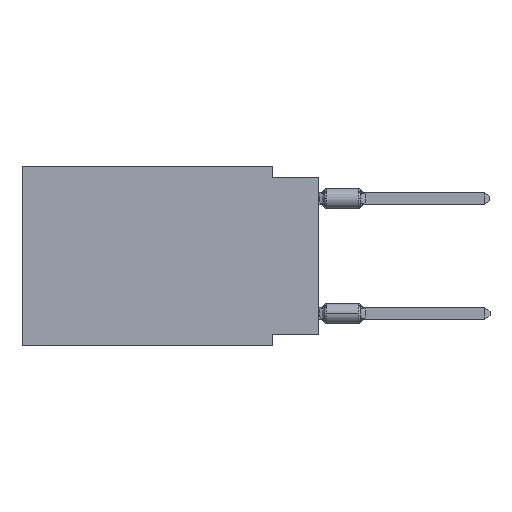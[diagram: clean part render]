
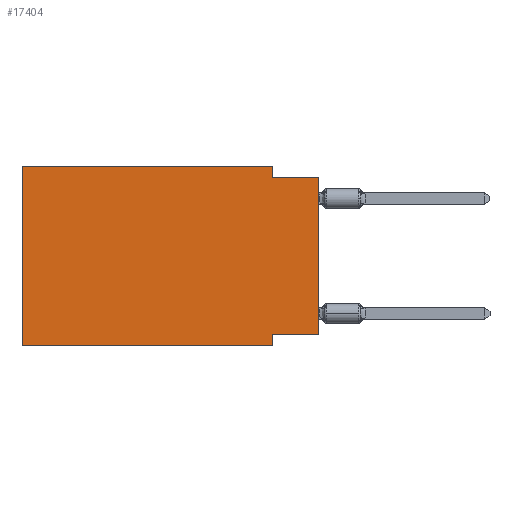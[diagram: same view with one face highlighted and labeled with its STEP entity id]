
A CAD part, left-side view. The second image highlights one B-rep face of the part: STEP entity #17404.
In plain terms, the highlighted planar face has unit normal (-1, 0, 0).
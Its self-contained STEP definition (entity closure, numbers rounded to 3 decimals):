
#373 = EDGE_CURVE ( 'NONE', #12863, #6835, #8443, .T. ) ;
#426 = VERTEX_POINT ( 'NONE', #7139 ) ;
#1110 = DIRECTION ( 'NONE',  ( 0., 0., 1. ) ) ;
#2010 = ORIENTED_EDGE ( 'NONE', *, *, #9848, .F. ) ;
#2150 = CARTESIAN_POINT ( 'NONE',  ( 0., 2.54, 0. ) ) ;
#3019 = ORIENTED_EDGE ( 'NONE', *, *, #11672, .F. ) ;
#4053 = LINE ( 'NONE', #6963, #6411 ) ;
#4659 = ORIENTED_EDGE ( 'NONE', *, *, #9476, .T. ) ;
#5147 = LINE ( 'NONE', #15395, #16175 ) ;
#5241 = DIRECTION ( 'NONE',  ( 0., -1., 0. ) ) ;
#5390 = EDGE_CURVE ( 'NONE', #8502, #426, #15495, .T. ) ;
#5392 = DIRECTION ( 'NONE',  ( 0., 0., 1. ) ) ;
#5429 = EDGE_CURVE ( 'NONE', #8502, #12863, #5147, .T. ) ;
#6411 = VECTOR ( 'NONE', #9880, 1000. ) ;
#6603 = LINE ( 'NONE', #12436, #9199 ) ;
#6703 = ORIENTED_EDGE ( 'NONE', *, *, #10009, .F. ) ;
#6835 = VERTEX_POINT ( 'NONE', #17760 ) ;
#6918 = CARTESIAN_POINT ( 'NONE',  ( 0., 0., -0.635 ) ) ;
#6963 = CARTESIAN_POINT ( 'NONE',  ( 0., 2.54, -9.906 ) ) ;
#6981 = ORIENTED_EDGE ( 'NONE', *, *, #5390, .T. ) ;
#7008 = FACE_OUTER_BOUND ( 'NONE', #15380, .T. ) ;
#7131 = VECTOR ( 'NONE', #10967, 1000. ) ;
#7139 = CARTESIAN_POINT ( 'NONE',  ( 0., 2.54, -9.906 ) ) ;
#7621 = VECTOR ( 'NONE', #8152, 1000. ) ;
#7835 = VERTEX_POINT ( 'NONE', #18274 ) ;
#7891 = VERTEX_POINT ( 'NONE', #8415 ) ;
#8152 = DIRECTION ( 'NONE',  ( 0., 0., -1. ) ) ;
#8221 = ORIENTED_EDGE ( 'NONE', *, *, #10196, .F. ) ;
#8415 = CARTESIAN_POINT ( 'NONE',  ( 0., 2.54, -9.271 ) ) ;
#8443 = LINE ( 'NONE', #14174, #7131 ) ;
#8502 = VERTEX_POINT ( 'NONE', #15122 ) ;
#9199 = VECTOR ( 'NONE', #5392, 1000. ) ;
#9476 = EDGE_CURVE ( 'NONE', #16156, #7835, #6603, .T. ) ;
#9646 = CARTESIAN_POINT ( 'NONE',  ( 0., 16.383, 0. ) ) ;
#9848 = EDGE_CURVE ( 'NONE', #16156, #7891, #16467, .T. ) ;
#9880 = DIRECTION ( 'NONE',  ( 0., 0., -1. ) ) ;
#10009 = EDGE_CURVE ( 'NONE', #7891, #426, #4053, .T. ) ;
#10018 = VECTOR ( 'NONE', #14070, 1000. ) ;
#10196 = EDGE_CURVE ( 'NONE', #16517, #7835, #13792, .T. ) ;
#10449 = VECTOR ( 'NONE', #5241, 1000. ) ;
#10967 = DIRECTION ( 'NONE',  ( 0., -1., 0. ) ) ;
#10990 = CARTESIAN_POINT ( 'NONE',  ( 0., 0., -9.271 ) ) ;
#11053 = ORIENTED_EDGE ( 'NONE', *, *, #5429, .F. ) ;
#11231 = CARTESIAN_POINT ( 'NONE',  ( 0., 16.383, -9.906 ) ) ;
#11318 = CARTESIAN_POINT ( 'NONE',  ( 0., 0., -9.271 ) ) ;
#11323 = PLANE ( 'NONE',  #12411 ) ;
#11672 = EDGE_CURVE ( 'NONE', #6835, #16517, #15029, .T. ) ;
#12411 = AXIS2_PLACEMENT_3D ( 'NONE', #17345, #12847, #17065 ) ;
#12436 = CARTESIAN_POINT ( 'NONE',  ( 0., 0., 0. ) ) ;
#12492 = VECTOR ( 'NONE', #18240, 1000. ) ;
#12847 = DIRECTION ( 'NONE',  ( 1., 0., 0. ) ) ;
#12863 = VERTEX_POINT ( 'NONE', #9646 ) ;
#13081 = CARTESIAN_POINT ( 'NONE',  ( 0., 2.54, -0.635 ) ) ;
#13792 = LINE ( 'NONE', #6918, #10018 ) ;
#13859 = ORIENTED_EDGE ( 'NONE', *, *, #373, .F. ) ;
#14070 = DIRECTION ( 'NONE',  ( 0., -1., 0. ) ) ;
#14174 = CARTESIAN_POINT ( 'NONE',  ( 0., 16.383, 0. ) ) ;
#15029 = LINE ( 'NONE', #2150, #7621 ) ;
#15122 = CARTESIAN_POINT ( 'NONE',  ( 0., 16.383, -9.906 ) ) ;
#15380 = EDGE_LOOP ( 'NONE', ( #4659, #8221, #3019, #13859, #11053, #6981, #6703, #2010 ) ) ;
#15395 = CARTESIAN_POINT ( 'NONE',  ( 0., 16.383, 0. ) ) ;
#15495 = LINE ( 'NONE', #11231, #10449 ) ;
#16156 = VERTEX_POINT ( 'NONE', #11318 ) ;
#16175 = VECTOR ( 'NONE', #1110, 1000. ) ;
#16467 = LINE ( 'NONE', #10990, #12492 ) ;
#16517 = VERTEX_POINT ( 'NONE', #13081 ) ;
#17065 = DIRECTION ( 'NONE',  ( 0., 0., -1. ) ) ;
#17345 = CARTESIAN_POINT ( 'NONE',  ( 0., 16.383, 0. ) ) ;
#17404 = ADVANCED_FACE ( 'NONE', ( #7008 ), #11323, .F. ) ;
#17760 = CARTESIAN_POINT ( 'NONE',  ( 0., 2.54, 0. ) ) ;
#18240 = DIRECTION ( 'NONE',  ( 0., 1., 0. ) ) ;
#18274 = CARTESIAN_POINT ( 'NONE',  ( 0., 0., -0.635 ) ) ;
